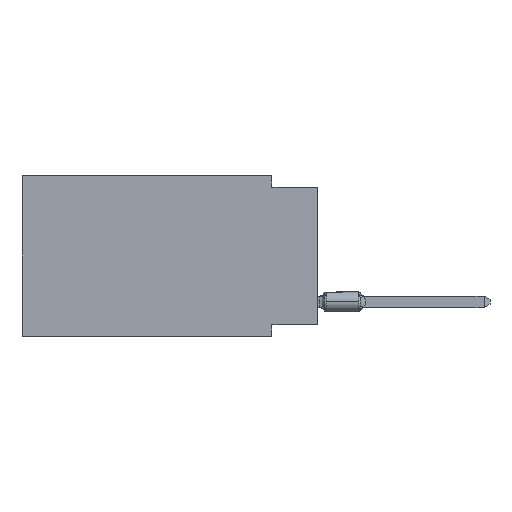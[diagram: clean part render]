
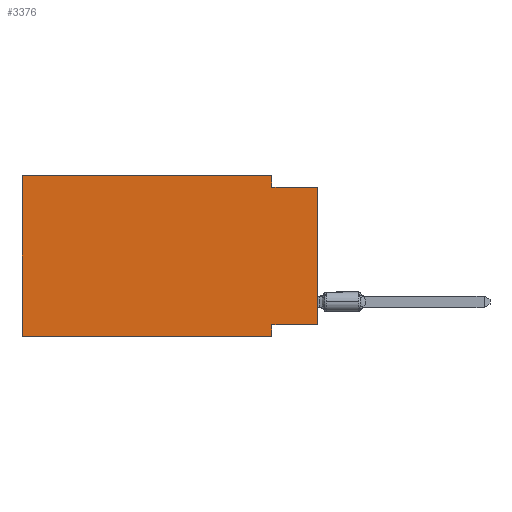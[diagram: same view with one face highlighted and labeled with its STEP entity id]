
A CAD part, left-side view. The second image highlights one B-rep face of the part: STEP entity #3376.
In plain terms, the highlighted planar face has unit normal (-1, 0, 0).
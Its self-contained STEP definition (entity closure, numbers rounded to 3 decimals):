
#70 = DIRECTION ( 'NONE',  ( 0., -1., 0. ) ) ;
#75 = CARTESIAN_POINT ( 'NONE',  ( 0., 2.54, 0. ) ) ;
#351 = EDGE_CURVE ( 'NONE', #15926, #6599, #14232, .T. ) ;
#812 = VERTEX_POINT ( 'NONE', #6358 ) ;
#821 = PLANE ( 'NONE',  #10972 ) ;
#1203 = DIRECTION ( 'NONE',  ( 0., 1., 0. ) ) ;
#1588 = LINE ( 'NONE', #20818, #7387 ) ;
#2550 = FACE_OUTER_BOUND ( 'NONE', #6022, .T. ) ;
#3055 = DIRECTION ( 'NONE',  ( 0., 0., -1. ) ) ;
#3376 = ADVANCED_FACE ( 'NONE', ( #2550 ), #821, .F. ) ;
#3436 = LINE ( 'NONE', #7132, #5351 ) ;
#3561 = VECTOR ( 'NONE', #18325, 1000. ) ;
#3658 = EDGE_CURVE ( 'NONE', #9500, #812, #8887, .T. ) ;
#3677 = CARTESIAN_POINT ( 'NONE',  ( 0., 16.383, 0. ) ) ;
#4233 = VECTOR ( 'NONE', #1203, 1000. ) ;
#4503 = EDGE_CURVE ( 'NONE', #8412, #4610, #4903, .T. ) ;
#4610 = VERTEX_POINT ( 'NONE', #14744 ) ;
#4903 = LINE ( 'NONE', #75, #7299 ) ;
#5351 = VECTOR ( 'NONE', #19443, 1000. ) ;
#5894 = DIRECTION ( 'NONE',  ( 1., 0., 0. ) ) ;
#6022 = EDGE_LOOP ( 'NONE', ( #7136, #16755, #13480, #14098, #14047, #12249, #17988, #17474 ) ) ;
#6358 = CARTESIAN_POINT ( 'NONE',  ( 0., 16.383, 0. ) ) ;
#6599 = VERTEX_POINT ( 'NONE', #13229 ) ;
#7132 = CARTESIAN_POINT ( 'NONE',  ( 0., 0., 0. ) ) ;
#7136 = ORIENTED_EDGE ( 'NONE', *, *, #21922, .T. ) ;
#7299 = VECTOR ( 'NONE', #3055, 1000. ) ;
#7387 = VECTOR ( 'NONE', #16165, 1000. ) ;
#7408 = DIRECTION ( 'NONE',  ( 0., 0., -1. ) ) ;
#8229 = EDGE_CURVE ( 'NONE', #812, #8412, #1588, .T. ) ;
#8412 = VERTEX_POINT ( 'NONE', #9385 ) ;
#8587 = CARTESIAN_POINT ( 'NONE',  ( 0., 16.383, -8.89 ) ) ;
#8887 = LINE ( 'NONE', #3677, #12887 ) ;
#9385 = CARTESIAN_POINT ( 'NONE',  ( 0., 2.54, 0. ) ) ;
#9500 = VERTEX_POINT ( 'NONE', #18263 ) ;
#10261 = CARTESIAN_POINT ( 'NONE',  ( 0., 2.54, -8.89 ) ) ;
#10425 = DIRECTION ( 'NONE',  ( 0., 0., -1. ) ) ;
#10500 = VECTOR ( 'NONE', #70, 1000. ) ;
#10887 = LINE ( 'NONE', #17899, #15612 ) ;
#10972 = AXIS2_PLACEMENT_3D ( 'NONE', #14853, #5894, #7408 ) ;
#12151 = EDGE_CURVE ( 'NONE', #4610, #21691, #13162, .T. ) ;
#12249 = ORIENTED_EDGE ( 'NONE', *, *, #21990, .T. ) ;
#12798 = CARTESIAN_POINT ( 'NONE',  ( 0., 0., -0.635 ) ) ;
#12887 = VECTOR ( 'NONE', #13829, 1000. ) ;
#13162 = LINE ( 'NONE', #22006, #3561 ) ;
#13229 = CARTESIAN_POINT ( 'NONE',  ( 0., 2.54, -8.255 ) ) ;
#13480 = ORIENTED_EDGE ( 'NONE', *, *, #4503, .F. ) ;
#13829 = DIRECTION ( 'NONE',  ( 0., 0., 1. ) ) ;
#14047 = ORIENTED_EDGE ( 'NONE', *, *, #3658, .F. ) ;
#14098 = ORIENTED_EDGE ( 'NONE', *, *, #8229, .F. ) ;
#14232 = LINE ( 'NONE', #16957, #4233 ) ;
#14744 = CARTESIAN_POINT ( 'NONE',  ( 0., 2.54, -0.635 ) ) ;
#14853 = CARTESIAN_POINT ( 'NONE',  ( 0., 16.383, 0. ) ) ;
#15612 = VECTOR ( 'NONE', #10425, 1000. ) ;
#15833 = LINE ( 'NONE', #8587, #10500 ) ;
#15926 = VERTEX_POINT ( 'NONE', #17632 ) ;
#16165 = DIRECTION ( 'NONE',  ( 0., -1., 0. ) ) ;
#16755 = ORIENTED_EDGE ( 'NONE', *, *, #12151, .F. ) ;
#16957 = CARTESIAN_POINT ( 'NONE',  ( 0., 0., -8.255 ) ) ;
#17474 = ORIENTED_EDGE ( 'NONE', *, *, #351, .F. ) ;
#17632 = CARTESIAN_POINT ( 'NONE',  ( 0., 0., -8.255 ) ) ;
#17899 = CARTESIAN_POINT ( 'NONE',  ( 0., 2.54, -8.89 ) ) ;
#17988 = ORIENTED_EDGE ( 'NONE', *, *, #21297, .F. ) ;
#18263 = CARTESIAN_POINT ( 'NONE',  ( 0., 16.383, -8.89 ) ) ;
#18325 = DIRECTION ( 'NONE',  ( 0., -1., 0. ) ) ;
#19443 = DIRECTION ( 'NONE',  ( 0., 0., 1. ) ) ;
#20818 = CARTESIAN_POINT ( 'NONE',  ( 0., 16.383, 0. ) ) ;
#21297 = EDGE_CURVE ( 'NONE', #6599, #21837, #10887, .T. ) ;
#21691 = VERTEX_POINT ( 'NONE', #12798 ) ;
#21837 = VERTEX_POINT ( 'NONE', #10261 ) ;
#21922 = EDGE_CURVE ( 'NONE', #15926, #21691, #3436, .T. ) ;
#21990 = EDGE_CURVE ( 'NONE', #9500, #21837, #15833, .T. ) ;
#22006 = CARTESIAN_POINT ( 'NONE',  ( 0., 0., -0.635 ) ) ;
